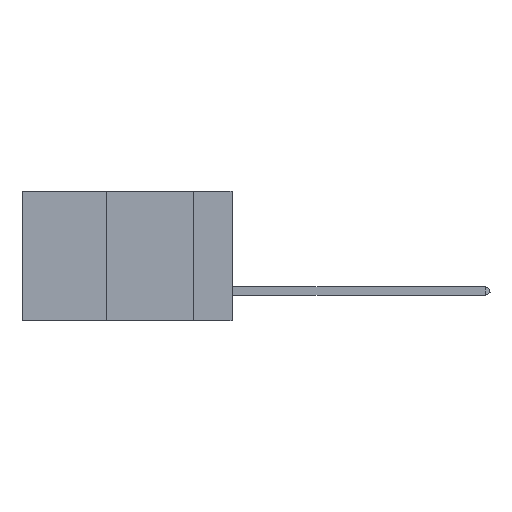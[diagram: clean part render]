
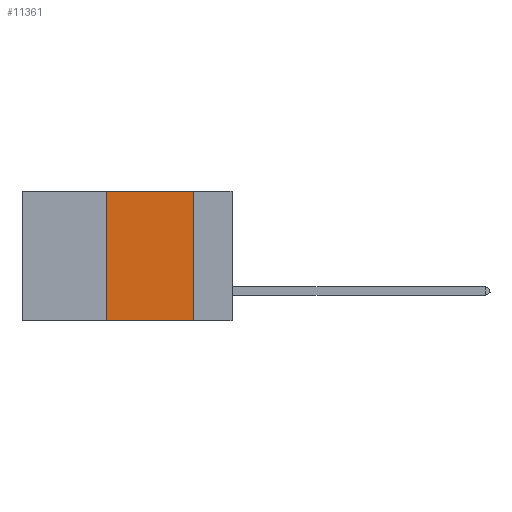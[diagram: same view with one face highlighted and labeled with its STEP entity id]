
A CAD part, left-side view. The second image highlights one B-rep face of the part: STEP entity #11361.
In plain terms, the highlighted planar face has unit normal (-1, 0, 0).
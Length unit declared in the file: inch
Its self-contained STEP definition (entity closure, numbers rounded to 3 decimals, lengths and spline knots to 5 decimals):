
#138 = VERTEX_POINT ( 'NONE', #9069 ) ;
#357 = DIRECTION ( 'NONE',  ( 0., -1., 0. ) ) ;
#454 = CARTESIAN_POINT ( 'NONE',  ( 0., 0.6, 0. ) ) ;
#1183 = VERTEX_POINT ( 'NONE', #3917 ) ;
#1586 = DIRECTION ( 'NONE',  ( 0., 0., 1. ) ) ;
#2168 = ORIENTED_EDGE ( 'NONE', *, *, #7139, .T. ) ;
#2202 = VECTOR ( 'NONE', #1586, 39.37008 ) ;
#2938 = CARTESIAN_POINT ( 'NONE',  ( 0., 0.6, -0.37 ) ) ;
#3145 = CARTESIAN_POINT ( 'NONE',  ( 0., 0.11, -0.37 ) ) ;
#3181 = VECTOR ( 'NONE', #357, 39.37008 ) ;
#3477 = CARTESIAN_POINT ( 'NONE',  ( 0., 0.6, 0. ) ) ;
#3917 = CARTESIAN_POINT ( 'NONE',  ( 0., 0.36, -0.37 ) ) ;
#4442 = LINE ( 'NONE', #3477, #3181 ) ;
#4586 = LINE ( 'NONE', #7650, #2202 ) ;
#4967 = EDGE_LOOP ( 'NONE', ( #6959, #6589, #6936, #2168 ) ) ;
#5731 = LINE ( 'NONE', #2938, #12583 ) ;
#5980 = VERTEX_POINT ( 'NONE', #8966 ) ;
#6084 = CARTESIAN_POINT ( 'NONE',  ( 0., 0.11, 0. ) ) ;
#6589 = ORIENTED_EDGE ( 'NONE', *, *, #13098, .F. ) ;
#6936 = ORIENTED_EDGE ( 'NONE', *, *, #8192, .F. ) ;
#6959 = ORIENTED_EDGE ( 'NONE', *, *, #11021, .F. ) ;
#7139 = EDGE_CURVE ( 'NONE', #1183, #10034, #5731, .T. ) ;
#7366 = VECTOR ( 'NONE', #10230, 39.37008 ) ;
#7527 = PLANE ( 'NONE',  #13162 ) ;
#7650 = CARTESIAN_POINT ( 'NONE',  ( 0., 0.36, 0. ) ) ;
#7658 = DIRECTION ( 'NONE',  ( 0., 0., -1. ) ) ;
#8192 = EDGE_CURVE ( 'NONE', #1183, #5980, #4586, .T. ) ;
#8966 = CARTESIAN_POINT ( 'NONE',  ( 0., 0.36, 0. ) ) ;
#9069 = CARTESIAN_POINT ( 'NONE',  ( 0., 0.11, 0. ) ) ;
#9249 = DIRECTION ( 'NONE',  ( 0., -1., 0. ) ) ;
#10034 = VERTEX_POINT ( 'NONE', #3145 ) ;
#10076 = FACE_OUTER_BOUND ( 'NONE', #4967, .T. ) ;
#10230 = DIRECTION ( 'NONE',  ( 0., 0., -1. ) ) ;
#10250 = LINE ( 'NONE', #6084, #7366 ) ;
#11021 = EDGE_CURVE ( 'NONE', #138, #10034, #10250, .T. ) ;
#11361 = ADVANCED_FACE ( 'NONE', ( #10076 ), #7527, .F. ) ;
#12583 = VECTOR ( 'NONE', #9249, 39.37008 ) ;
#12716 = DIRECTION ( 'NONE',  ( 1., 0., 0. ) ) ;
#13098 = EDGE_CURVE ( 'NONE', #5980, #138, #4442, .T. ) ;
#13162 = AXIS2_PLACEMENT_3D ( 'NONE', #454, #12716, #7658 ) ;
